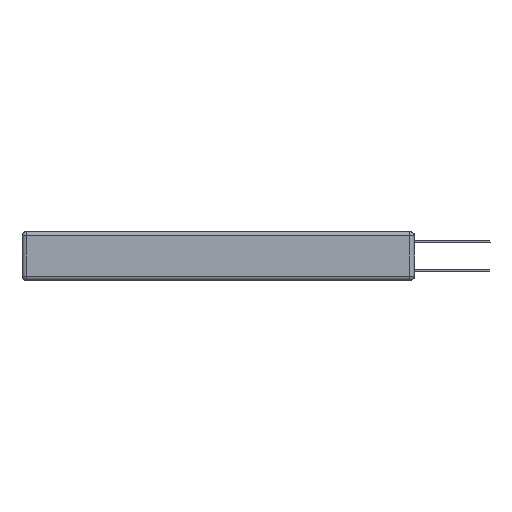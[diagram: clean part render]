
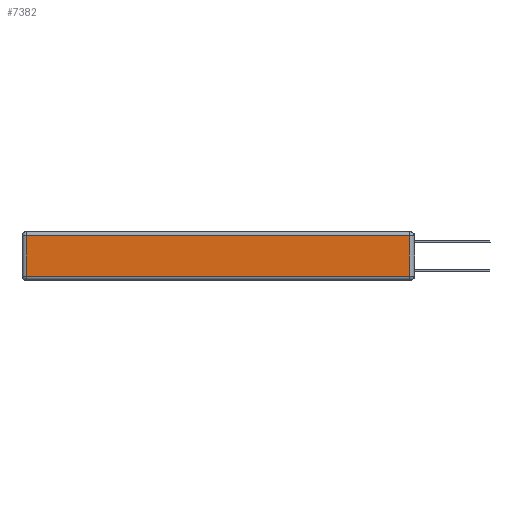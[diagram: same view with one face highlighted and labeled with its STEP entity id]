
A CAD part, left-side view. The second image highlights one B-rep face of the part: STEP entity #7382.
In plain terms, the highlighted planar face has unit normal (-1, 0, 0).
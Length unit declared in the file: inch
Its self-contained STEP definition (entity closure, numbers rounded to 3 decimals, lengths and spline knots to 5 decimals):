
#60 = CARTESIAN_POINT ( 'NONE',  ( 0., 2.75, -0.03 ) ) ;
#1341 = CARTESIAN_POINT ( 'NONE',  ( 0., 0.03, -0.03 ) ) ;
#1701 = CARTESIAN_POINT ( 'NONE',  ( 0., 0.03, -0.313 ) ) ;
#1716 = DIRECTION ( 'NONE',  ( 0., 1., 0. ) ) ;
#2316 = VERTEX_POINT ( 'NONE', #4832 ) ;
#2501 = VECTOR ( 'NONE', #10612, 39.37008 ) ;
#3763 = EDGE_CURVE ( 'NONE', #14386, #2316, #10647, .T. ) ;
#4263 = DIRECTION ( 'NONE',  ( -1., 0., 0. ) ) ;
#4816 = ORIENTED_EDGE ( 'NONE', *, *, #17559, .T. ) ;
#4832 = CARTESIAN_POINT ( 'NONE',  ( 0., 2.72, -0.03 ) ) ;
#4876 = CARTESIAN_POINT ( 'NONE',  ( 0., 0., -0.313 ) ) ;
#5010 = EDGE_LOOP ( 'NONE', ( #14254, #4816, #15662, #18311 ) ) ;
#5122 = CARTESIAN_POINT ( 'NONE',  ( 0., 2.72, -0.313 ) ) ;
#7382 = ADVANCED_FACE ( 'NONE', ( #13101 ), #7559, .T. ) ;
#7559 = PLANE ( 'NONE',  #10605 ) ;
#8891 = VECTOR ( 'NONE', #18458, 39.37008 ) ;
#9668 = LINE ( 'NONE', #11888, #8891 ) ;
#9898 = VECTOR ( 'NONE', #19999, 39.37008 ) ;
#10372 = VERTEX_POINT ( 'NONE', #1701 ) ;
#10605 = AXIS2_PLACEMENT_3D ( 'NONE', #21116, #4263, #12592 ) ;
#10612 = DIRECTION ( 'NONE',  ( 0., 0., -1. ) ) ;
#10647 = LINE ( 'NONE', #60, #11175 ) ;
#11175 = VECTOR ( 'NONE', #1716, 39.37008 ) ;
#11603 = EDGE_CURVE ( 'NONE', #13367, #10372, #20689, .T. ) ;
#11888 = CARTESIAN_POINT ( 'NONE',  ( 0., 0.03, -0.343 ) ) ;
#12592 = DIRECTION ( 'NONE',  ( 0., 0., 1. ) ) ;
#12846 = EDGE_CURVE ( 'NONE', #2316, #13367, #16154, .T. ) ;
#13101 = FACE_OUTER_BOUND ( 'NONE', #5010, .T. ) ;
#13367 = VERTEX_POINT ( 'NONE', #5122 ) ;
#14053 = CARTESIAN_POINT ( 'NONE',  ( 0., 2.72, -0.343 ) ) ;
#14254 = ORIENTED_EDGE ( 'NONE', *, *, #11603, .T. ) ;
#14386 = VERTEX_POINT ( 'NONE', #1341 ) ;
#15662 = ORIENTED_EDGE ( 'NONE', *, *, #3763, .T. ) ;
#16154 = LINE ( 'NONE', #14053, #2501 ) ;
#17559 = EDGE_CURVE ( 'NONE', #10372, #14386, #9668, .T. ) ;
#18311 = ORIENTED_EDGE ( 'NONE', *, *, #12846, .T. ) ;
#18458 = DIRECTION ( 'NONE',  ( 0., 0., 1. ) ) ;
#19999 = DIRECTION ( 'NONE',  ( 0., -1., 0. ) ) ;
#20689 = LINE ( 'NONE', #4876, #9898 ) ;
#21116 = CARTESIAN_POINT ( 'NONE',  ( 0., 0., -0.343 ) ) ;
